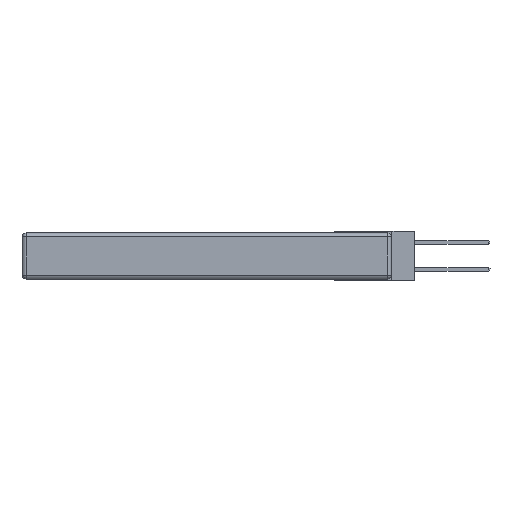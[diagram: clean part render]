
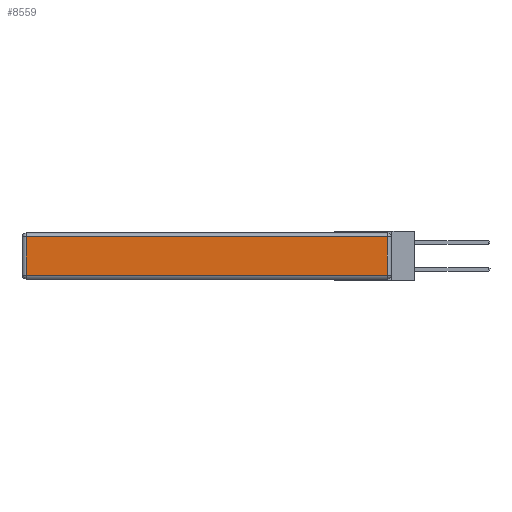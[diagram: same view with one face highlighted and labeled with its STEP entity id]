
A CAD part, left-side view. The second image highlights one B-rep face of the part: STEP entity #8559.
In plain terms, the highlighted planar face has unit normal (-1, 0, 0).
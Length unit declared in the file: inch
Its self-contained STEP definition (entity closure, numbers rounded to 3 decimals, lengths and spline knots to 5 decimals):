
#746 = ORIENTED_EDGE ( 'NONE', *, *, #8079, .T. ) ;
#1168 = VERTEX_POINT ( 'NONE', #6608 ) ;
#1284 = VECTOR ( 'NONE', #6256, 39.37008 ) ;
#2221 = LINE ( 'NONE', #12744, #13369 ) ;
#2346 = EDGE_CURVE ( 'NONE', #2960, #10599, #2221, .T. ) ;
#2923 = CARTESIAN_POINT ( 'NONE',  ( 0., 0., -0.343 ) ) ;
#2960 = VERTEX_POINT ( 'NONE', #12757 ) ;
#2967 = PLANE ( 'NONE',  #13355 ) ;
#3145 = LINE ( 'NONE', #5370, #3968 ) ;
#3193 = CARTESIAN_POINT ( 'NONE',  ( 0., 0., -0.313 ) ) ;
#3968 = VECTOR ( 'NONE', #9542, 39.37008 ) ;
#5012 = EDGE_CURVE ( 'NONE', #10599, #1168, #10593, .T. ) ;
#5316 = LINE ( 'NONE', #8209, #11544 ) ;
#5370 = CARTESIAN_POINT ( 'NONE',  ( 0., 2.75, -0.03 ) ) ;
#5979 = DIRECTION ( 'NONE',  ( -1., 0., 0. ) ) ;
#6100 = ORIENTED_EDGE ( 'NONE', *, *, #2346, .T. ) ;
#6256 = DIRECTION ( 'NONE',  ( 0., -1., 0. ) ) ;
#6608 = CARTESIAN_POINT ( 'NONE',  ( 0., 0.03, -0.313 ) ) ;
#7014 = ORIENTED_EDGE ( 'NONE', *, *, #12657, .T. ) ;
#7269 = CARTESIAN_POINT ( 'NONE',  ( 0., 0.03, -0.03 ) ) ;
#7533 = DIRECTION ( 'NONE',  ( 0., 0., -1. ) ) ;
#8036 = VERTEX_POINT ( 'NONE', #7269 ) ;
#8079 = EDGE_CURVE ( 'NONE', #8036, #2960, #3145, .T. ) ;
#8209 = CARTESIAN_POINT ( 'NONE',  ( 0., 0.03, -0.343 ) ) ;
#8559 = ADVANCED_FACE ( 'NONE', ( #10671 ), #2967, .T. ) ;
#9542 = DIRECTION ( 'NONE',  ( 0., 1., 0. ) ) ;
#10249 = ORIENTED_EDGE ( 'NONE', *, *, #5012, .T. ) ;
#10593 = LINE ( 'NONE', #3193, #1284 ) ;
#10599 = VERTEX_POINT ( 'NONE', #11540 ) ;
#10671 = FACE_OUTER_BOUND ( 'NONE', #11383, .T. ) ;
#11383 = EDGE_LOOP ( 'NONE', ( #10249, #7014, #746, #6100 ) ) ;
#11396 = DIRECTION ( 'NONE',  ( 0., 0., 1. ) ) ;
#11540 = CARTESIAN_POINT ( 'NONE',  ( 0., 2.72, -0.313 ) ) ;
#11544 = VECTOR ( 'NONE', #12555, 39.37008 ) ;
#12555 = DIRECTION ( 'NONE',  ( 0., 0., 1. ) ) ;
#12657 = EDGE_CURVE ( 'NONE', #1168, #8036, #5316, .T. ) ;
#12744 = CARTESIAN_POINT ( 'NONE',  ( 0., 2.72, -0.343 ) ) ;
#12757 = CARTESIAN_POINT ( 'NONE',  ( 0., 2.72, -0.03 ) ) ;
#13355 = AXIS2_PLACEMENT_3D ( 'NONE', #2923, #5979, #11396 ) ;
#13369 = VECTOR ( 'NONE', #7533, 39.37008 ) ;
